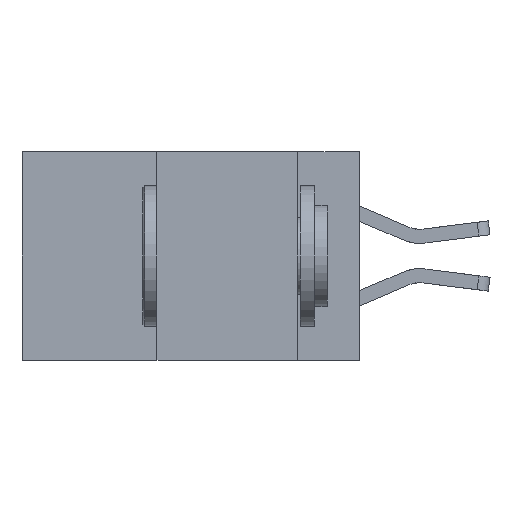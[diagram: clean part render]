
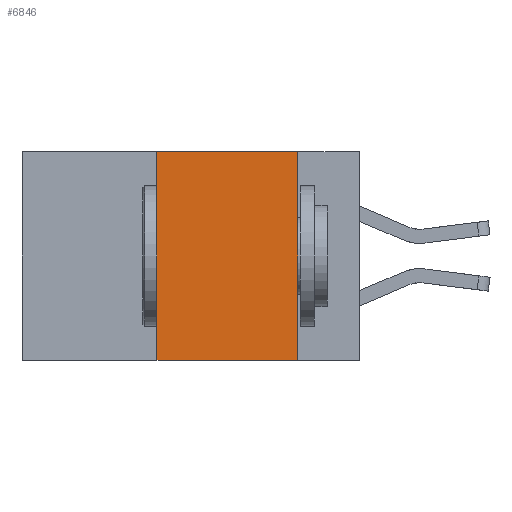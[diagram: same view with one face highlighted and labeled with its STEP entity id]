
A CAD part, left-side view. The second image highlights one B-rep face of the part: STEP entity #6846.
In plain terms, the highlighted planar face has unit normal (-1, 0, 0).
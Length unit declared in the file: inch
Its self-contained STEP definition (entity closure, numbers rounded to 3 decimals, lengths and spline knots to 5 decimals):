
#83 = CARTESIAN_POINT ( 'NONE',  ( 0., 0.6, 0. ) ) ;
#198 = LINE ( 'NONE', #11939, #12531 ) ;
#290 = CARTESIAN_POINT ( 'NONE',  ( 0., 0.11, -0.37 ) ) ;
#995 = ORIENTED_EDGE ( 'NONE', *, *, #10575, .F. ) ;
#2248 = EDGE_LOOP ( 'NONE', ( #10887, #3597, #995, #3957 ) ) ;
#2425 = DIRECTION ( 'NONE',  ( 0., 0., 1. ) ) ;
#2614 = DIRECTION ( 'NONE',  ( 0., 0., -1. ) ) ;
#2659 = DIRECTION ( 'NONE',  ( 1., 0., 0. ) ) ;
#2680 = AXIS2_PLACEMENT_3D ( 'NONE', #83, #2659, #2614 ) ;
#2687 = PLANE ( 'NONE',  #2680 ) ;
#2981 = LINE ( 'NONE', #11709, #5548 ) ;
#3335 = DIRECTION ( 'NONE',  ( 0., 0., -1. ) ) ;
#3445 = EDGE_CURVE ( 'NONE', #5302, #3461, #5016, .T. ) ;
#3461 = VERTEX_POINT ( 'NONE', #290 ) ;
#3597 = ORIENTED_EDGE ( 'NONE', *, *, #10641, .F. ) ;
#3957 = ORIENTED_EDGE ( 'NONE', *, *, #11059, .T. ) ;
#4254 = FACE_OUTER_BOUND ( 'NONE', #2248, .T. ) ;
#5016 = LINE ( 'NONE', #5861, #7293 ) ;
#5059 = LINE ( 'NONE', #6634, #10012 ) ;
#5302 = VERTEX_POINT ( 'NONE', #6071 ) ;
#5548 = VECTOR ( 'NONE', #7306, 39.37008 ) ;
#5861 = CARTESIAN_POINT ( 'NONE',  ( 0., 0.11, 0. ) ) ;
#6071 = CARTESIAN_POINT ( 'NONE',  ( 0., 0.11, 0. ) ) ;
#6634 = CARTESIAN_POINT ( 'NONE',  ( 0., 0.6, 0. ) ) ;
#6846 = ADVANCED_FACE ( 'NONE', ( #4254 ), #2687, .F. ) ;
#7135 = VERTEX_POINT ( 'NONE', #10168 ) ;
#7293 = VECTOR ( 'NONE', #3335, 39.37008 ) ;
#7306 = DIRECTION ( 'NONE',  ( 0., -1., 0. ) ) ;
#8387 = CARTESIAN_POINT ( 'NONE',  ( 0., 0.36, -0.37 ) ) ;
#9645 = VERTEX_POINT ( 'NONE', #8387 ) ;
#10012 = VECTOR ( 'NONE', #12007, 39.37008 ) ;
#10168 = CARTESIAN_POINT ( 'NONE',  ( 0., 0.36, 0. ) ) ;
#10575 = EDGE_CURVE ( 'NONE', #9645, #7135, #198, .T. ) ;
#10641 = EDGE_CURVE ( 'NONE', #7135, #5302, #5059, .T. ) ;
#10887 = ORIENTED_EDGE ( 'NONE', *, *, #3445, .F. ) ;
#11059 = EDGE_CURVE ( 'NONE', #9645, #3461, #2981, .T. ) ;
#11709 = CARTESIAN_POINT ( 'NONE',  ( 0., 0.6, -0.37 ) ) ;
#11939 = CARTESIAN_POINT ( 'NONE',  ( 0., 0.36, 0. ) ) ;
#12007 = DIRECTION ( 'NONE',  ( 0., -1., 0. ) ) ;
#12531 = VECTOR ( 'NONE', #2425, 39.37008 ) ;
